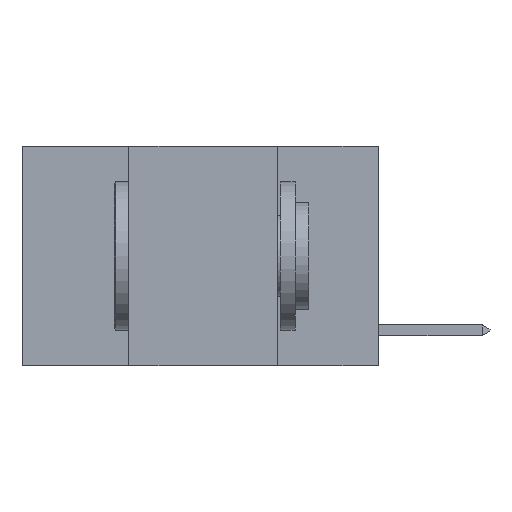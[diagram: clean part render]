
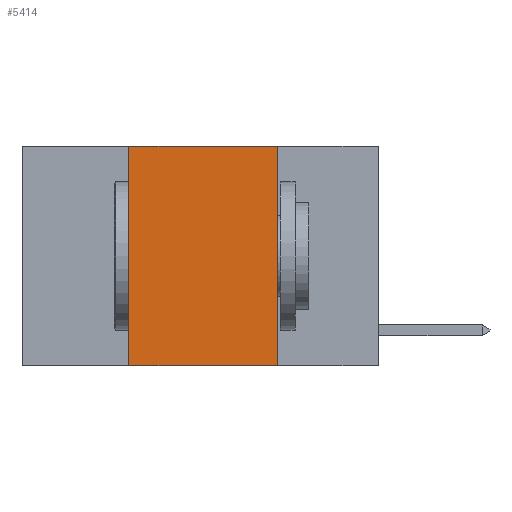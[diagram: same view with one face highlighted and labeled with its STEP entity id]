
A CAD part, left-side view. The second image highlights one B-rep face of the part: STEP entity #5414.
In plain terms, the highlighted planar face has unit normal (-1, 0, 0).
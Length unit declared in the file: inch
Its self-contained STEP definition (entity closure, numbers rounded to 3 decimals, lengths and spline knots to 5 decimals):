
#92 = VERTEX_POINT ( 'NONE', #15704 ) ;
#412 = CARTESIAN_POINT ( 'NONE',  ( 0., 0.42, -0.37 ) ) ;
#468 = VERTEX_POINT ( 'NONE', #2608 ) ;
#2403 = LINE ( 'NONE', #14244, #11656 ) ;
#2404 = VECTOR ( 'NONE', #5533, 39.37008 ) ;
#2608 = CARTESIAN_POINT ( 'NONE',  ( 0., 0.17, -0.37 ) ) ;
#3291 = ORIENTED_EDGE ( 'NONE', *, *, #11644, .F. ) ;
#3669 = ORIENTED_EDGE ( 'NONE', *, *, #7451, .T. ) ;
#3764 = CARTESIAN_POINT ( 'NONE',  ( 0., 0.17, 0. ) ) ;
#4256 = EDGE_CURVE ( 'NONE', #6536, #92, #6569, .T. ) ;
#4671 = PLANE ( 'NONE',  #15483 ) ;
#5414 = ADVANCED_FACE ( 'NONE', ( #12283 ), #4671, .F. ) ;
#5533 = DIRECTION ( 'NONE',  ( 0., -1., 0. ) ) ;
#5670 = LINE ( 'NONE', #9828, #2404 ) ;
#5908 = DIRECTION ( 'NONE',  ( 0., 0., -1. ) ) ;
#5939 = CARTESIAN_POINT ( 'NONE',  ( 0., 0.6, 0. ) ) ;
#6190 = ORIENTED_EDGE ( 'NONE', *, *, #6701, .F. ) ;
#6536 = VERTEX_POINT ( 'NONE', #14260 ) ;
#6569 = LINE ( 'NONE', #5939, #9336 ) ;
#6701 = EDGE_CURVE ( 'NONE', #92, #468, #13376, .T. ) ;
#7451 = EDGE_CURVE ( 'NONE', #13413, #468, #5670, .T. ) ;
#7825 = VECTOR ( 'NONE', #12184, 39.37008 ) ;
#9279 = EDGE_LOOP ( 'NONE', ( #6190, #12510, #3291, #3669 ) ) ;
#9336 = VECTOR ( 'NONE', #13085, 39.37008 ) ;
#9828 = CARTESIAN_POINT ( 'NONE',  ( 0., 0.6, -0.37 ) ) ;
#10555 = DIRECTION ( 'NONE',  ( 0., 0., 1. ) ) ;
#11644 = EDGE_CURVE ( 'NONE', #13413, #6536, #2403, .T. ) ;
#11656 = VECTOR ( 'NONE', #10555, 39.37008 ) ;
#11838 = CARTESIAN_POINT ( 'NONE',  ( 0., 0.6, 0. ) ) ;
#12184 = DIRECTION ( 'NONE',  ( 0., 0., -1. ) ) ;
#12283 = FACE_OUTER_BOUND ( 'NONE', #9279, .T. ) ;
#12510 = ORIENTED_EDGE ( 'NONE', *, *, #4256, .F. ) ;
#13058 = DIRECTION ( 'NONE',  ( 1., 0., 0. ) ) ;
#13085 = DIRECTION ( 'NONE',  ( 0., -1., 0. ) ) ;
#13376 = LINE ( 'NONE', #3764, #7825 ) ;
#13413 = VERTEX_POINT ( 'NONE', #412 ) ;
#14244 = CARTESIAN_POINT ( 'NONE',  ( 0., 0.42, 0. ) ) ;
#14260 = CARTESIAN_POINT ( 'NONE',  ( 0., 0.42, 0. ) ) ;
#15483 = AXIS2_PLACEMENT_3D ( 'NONE', #11838, #13058, #5908 ) ;
#15704 = CARTESIAN_POINT ( 'NONE',  ( 0., 0.17, 0. ) ) ;
